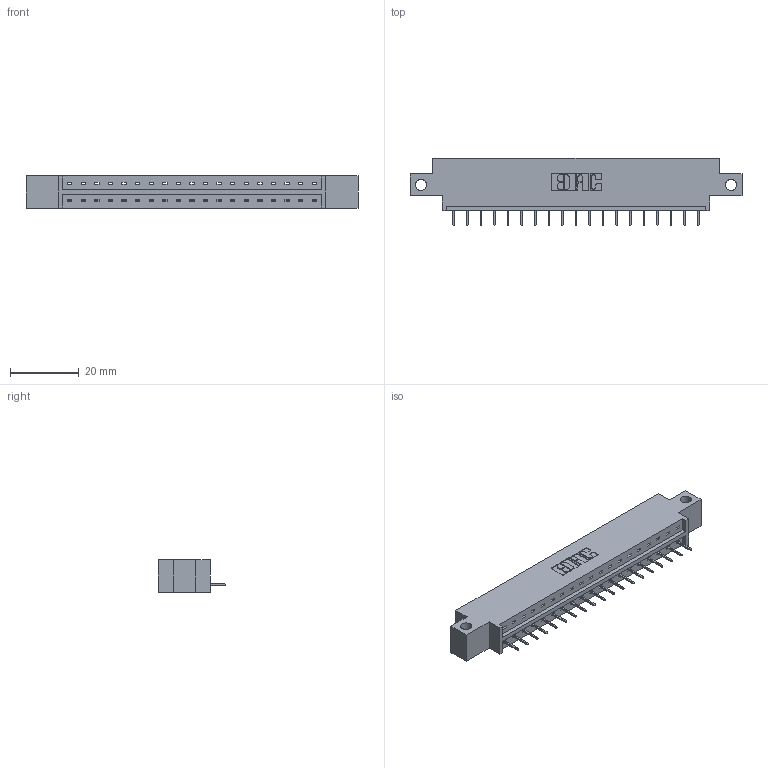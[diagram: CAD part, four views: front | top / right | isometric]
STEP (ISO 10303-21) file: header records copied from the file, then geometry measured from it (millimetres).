
FILE_DESCRIPTION (( 'STEP AP203' ), '1' );
FILE_NAME ('833-019-524-612.STEP', '2020-06-01T00:22:16', ( '' ), ( '' ), 'SwSTEP 2.0', 'SolidWorks 2020', '' );
FILE_SCHEMA (( 'CONFIG_CONTROL_DESIGN' ));
Length unit declared in the file: inch
Products named in the file (3): 833 Part_Offset - Side; 833-019-524-612; 345-292-001_345-293-124
Assembly tree (20 placements, depth 2):
  833-019-524-612
    833 Part_Offset - Side
    345-292-001_345-293-124  x19
Bounding box: 96.82 x 19.69 x 9.4 mm (x, y, z)
Volume: 9155.4 mm3; surface area: 9540.2 mm2
Topology: 20 solids, 20 shells, 1296 faces, 3743 edges, 2418 vertices
Faces by surface type: plane 986, cylinder 310
Entity records: 14799 total; most frequent: CARTESIAN_POINT 2563, ORIENTED_EDGE 2518, DIRECTION 2209, EDGE_CURVE 1259, VECTOR 1135, LINE 1135, VERTEX_POINT 834, AXIS2_PLACEMENT_3D 537
